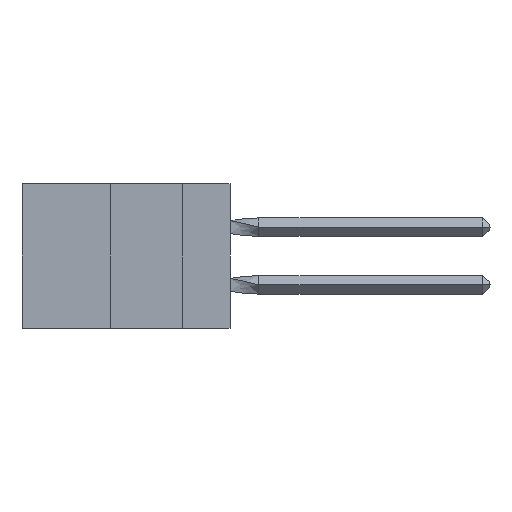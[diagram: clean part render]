
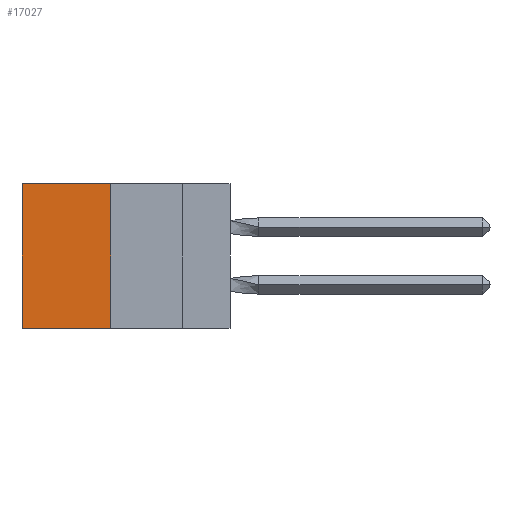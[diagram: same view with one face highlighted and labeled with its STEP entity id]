
A CAD part, left-side view. The second image highlights one B-rep face of the part: STEP entity #17027.
In plain terms, the highlighted planar face has unit normal (-1, 0, 0).
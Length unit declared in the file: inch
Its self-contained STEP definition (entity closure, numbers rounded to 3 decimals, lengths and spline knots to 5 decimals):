
#350 = VERTEX_POINT ( 'NONE', #19895 ) ;
#1106 = VERTEX_POINT ( 'NONE', #5374 ) ;
#1230 = VECTOR ( 'NONE', #9113, 39.37008 ) ;
#1265 = CARTESIAN_POINT ( 'NONE',  ( 0.305, 0.72, -0.5 ) ) ;
#1543 = ORIENTED_EDGE ( 'NONE', *, *, #15254, .T. ) ;
#2259 = EDGE_CURVE ( 'NONE', #350, #17132, #19088, .T. ) ;
#2474 = CARTESIAN_POINT ( 'NONE',  ( 0.305, 0.413, -0.5 ) ) ;
#2519 = LINE ( 'NONE', #2474, #1230 ) ;
#3404 = CARTESIAN_POINT ( 'NONE',  ( 0.305, 0.72, 0. ) ) ;
#4643 = EDGE_LOOP ( 'NONE', ( #1543, #4742, #21066, #9401 ) ) ;
#4742 = ORIENTED_EDGE ( 'NONE', *, *, #6657, .F. ) ;
#5041 = DIRECTION ( 'NONE',  ( 0., 0., -1. ) ) ;
#5374 = CARTESIAN_POINT ( 'NONE',  ( 0.305, 0.413, -0.5 ) ) ;
#5608 = DIRECTION ( 'NONE',  ( 0., 0., -1. ) ) ;
#6657 = EDGE_CURVE ( 'NONE', #1106, #8219, #2519, .T. ) ;
#7270 = CARTESIAN_POINT ( 'NONE',  ( 0.305, 0.72, -0.5 ) ) ;
#8219 = VERTEX_POINT ( 'NONE', #1265 ) ;
#8530 = VECTOR ( 'NONE', #11921, 39.37008 ) ;
#9113 = DIRECTION ( 'NONE',  ( 0., 1., 0. ) ) ;
#9401 = ORIENTED_EDGE ( 'NONE', *, *, #2259, .T. ) ;
#9621 = LINE ( 'NONE', #7270, #18447 ) ;
#9979 = DIRECTION ( 'NONE',  ( 0., 1., 0. ) ) ;
#10279 = CARTESIAN_POINT ( 'NONE',  ( 0.305, 0.413, -0.5 ) ) ;
#10637 = EDGE_CURVE ( 'NONE', #350, #1106, #17858, .T. ) ;
#11586 = PLANE ( 'NONE',  #18211 ) ;
#11921 = DIRECTION ( 'NONE',  ( 0., 0., -1. ) ) ;
#13233 = CARTESIAN_POINT ( 'NONE',  ( 0.305, 0.413, -0.5 ) ) ;
#13583 = VECTOR ( 'NONE', #9979, 39.37008 ) ;
#14928 = DIRECTION ( 'NONE',  ( 1., 0., 0. ) ) ;
#15183 = CARTESIAN_POINT ( 'NONE',  ( 0.305, 0.413, 0. ) ) ;
#15254 = EDGE_CURVE ( 'NONE', #17132, #8219, #9621, .T. ) ;
#17027 = ADVANCED_FACE ( 'NONE', ( #19429 ), #11586, .F. ) ;
#17132 = VERTEX_POINT ( 'NONE', #3404 ) ;
#17858 = LINE ( 'NONE', #10279, #8530 ) ;
#18211 = AXIS2_PLACEMENT_3D ( 'NONE', #13233, #14928, #5041 ) ;
#18447 = VECTOR ( 'NONE', #5608, 39.37008 ) ;
#19088 = LINE ( 'NONE', #15183, #13583 ) ;
#19429 = FACE_OUTER_BOUND ( 'NONE', #4643, .T. ) ;
#19895 = CARTESIAN_POINT ( 'NONE',  ( 0.305, 0.413, 0. ) ) ;
#21066 = ORIENTED_EDGE ( 'NONE', *, *, #10637, .F. ) ;
